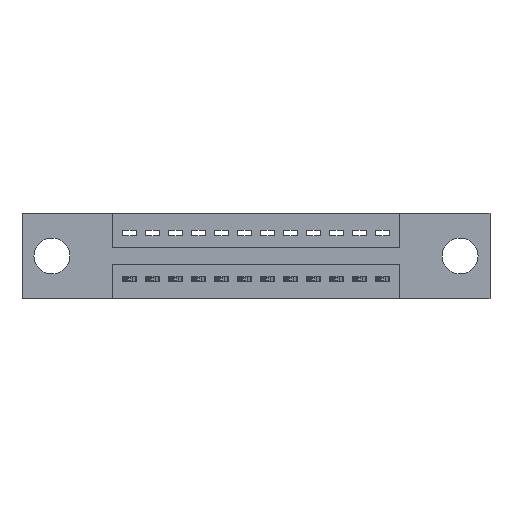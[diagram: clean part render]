
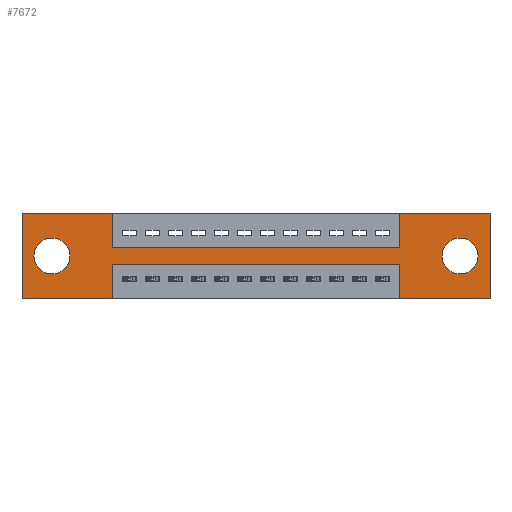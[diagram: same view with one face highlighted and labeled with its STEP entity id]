
A CAD part, front view. The second image highlights one B-rep face of the part: STEP entity #7672.
In plain terms, the highlighted planar face has unit normal (0, -1, 0).
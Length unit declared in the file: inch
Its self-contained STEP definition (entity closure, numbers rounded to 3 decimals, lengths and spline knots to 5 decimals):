
#318 = ORIENTED_EDGE ( 'NONE', *, *, #12914, .F. ) ;
#356 = VECTOR ( 'NONE', #7961, 39.37008 ) ;
#487 = EDGE_CURVE ( 'NONE', #9117, #1212, #12375, .T. ) ;
#604 = DIRECTION ( 'NONE',  ( -1., 0., 0. ) ) ;
#720 = ORIENTED_EDGE ( 'NONE', *, *, #12855, .F. ) ;
#855 = EDGE_CURVE ( 'NONE', #6111, #11537, #11433, .T. ) ;
#1012 = VECTOR ( 'NONE', #604, 39.37008 ) ;
#1043 = PLANE ( 'NONE',  #3110 ) ;
#1212 = VERTEX_POINT ( 'NONE', #1814 ) ;
#1356 = VECTOR ( 'NONE', #6458, 39.37008 ) ;
#1400 = DIRECTION ( 'NONE',  ( 0., 1., 0. ) ) ;
#1408 = ORIENTED_EDGE ( 'NONE', *, *, #5395, .F. ) ;
#1462 = CARTESIAN_POINT ( 'NONE',  ( 0., 0., 0. ) ) ;
#1665 = DIRECTION ( 'NONE',  ( 1., 0., 0. ) ) ;
#1699 = VECTOR ( 'NONE', #12983, 39.37008 ) ;
#1769 = EDGE_LOOP ( 'NONE', ( #11584, #6691 ) ) ;
#1786 = CARTESIAN_POINT ( 'NONE',  ( 1.6425, 0., 0. ) ) ;
#1814 = CARTESIAN_POINT ( 'NONE',  ( 1.6425, 0., -0.22 ) ) ;
#1876 = CARTESIAN_POINT ( 'NONE',  ( 1.905, 0., -0.263 ) ) ;
#1908 = VERTEX_POINT ( 'NONE', #6651 ) ;
#2068 = CARTESIAN_POINT ( 'NONE',  ( 0., 0., -0.37 ) ) ;
#2080 = EDGE_CURVE ( 'NONE', #7362, #10006, #7179, .T. ) ;
#2189 = CIRCLE ( 'NONE', #7160, 0.078 ) ;
#2197 = ORIENTED_EDGE ( 'NONE', *, *, #4360, .F. ) ;
#2454 = LINE ( 'NONE', #3017, #1699 ) ;
#2482 = EDGE_CURVE ( 'NONE', #6165, #11500, #4491, .T. ) ;
#2590 = EDGE_LOOP ( 'NONE', ( #10549, #720, #6742, #1408, #318, #6607, #2197, #4417, #5114, #8214, #8763, #4503 ) ) ;
#2599 = CARTESIAN_POINT ( 'NONE',  ( 0.13, 0., -0.107 ) ) ;
#2785 = DIRECTION ( 'NONE',  ( 0., 0., 1. ) ) ;
#2831 = DIRECTION ( 'NONE',  ( 0., 1., 0. ) ) ;
#2920 = VERTEX_POINT ( 'NONE', #3381 ) ;
#3017 = CARTESIAN_POINT ( 'NONE',  ( 0.3925, 0., -0.37 ) ) ;
#3110 = AXIS2_PLACEMENT_3D ( 'NONE', #2068, #6134, #8131 ) ;
#3120 = AXIS2_PLACEMENT_3D ( 'NONE', #12796, #2831, #2785 ) ;
#3379 = FACE_OUTER_BOUND ( 'NONE', #2590, .T. ) ;
#3381 = CARTESIAN_POINT ( 'NONE',  ( 2.035, 0., -0.37 ) ) ;
#3842 = ORIENTED_EDGE ( 'NONE', *, *, #10488, .T. ) ;
#3873 = VECTOR ( 'NONE', #1665, 39.37008 ) ;
#3937 = DIRECTION ( 'NONE',  ( 0., 0., -1. ) ) ;
#4031 = CARTESIAN_POINT ( 'NONE',  ( 0.3925, 0., -0.22 ) ) ;
#4063 = EDGE_CURVE ( 'NONE', #4259, #1908, #7414, .T. ) ;
#4072 = CARTESIAN_POINT ( 'NONE',  ( 2.035, 0., 0. ) ) ;
#4089 = CARTESIAN_POINT ( 'NONE',  ( 0., 0., -0.37 ) ) ;
#4112 = LINE ( 'NONE', #12458, #1356 ) ;
#4259 = VERTEX_POINT ( 'NONE', #6526 ) ;
#4360 = EDGE_CURVE ( 'NONE', #11500, #7362, #11028, .T. ) ;
#4417 = ORIENTED_EDGE ( 'NONE', *, *, #2482, .F. ) ;
#4491 = LINE ( 'NONE', #12496, #3873 ) ;
#4503 = ORIENTED_EDGE ( 'NONE', *, *, #6720, .F. ) ;
#4535 = LINE ( 'NONE', #4072, #10818 ) ;
#4577 = CARTESIAN_POINT ( 'NONE',  ( 2.035, 0., 0. ) ) ;
#4677 = AXIS2_PLACEMENT_3D ( 'NONE', #5333, #1400, #12327 ) ;
#4707 = DIRECTION ( 'NONE',  ( 0., 0., 1. ) ) ;
#4844 = EDGE_CURVE ( 'NONE', #11537, #6111, #2189, .T. ) ;
#4854 = LINE ( 'NONE', #4031, #356 ) ;
#4955 = CARTESIAN_POINT ( 'NONE',  ( 0.13, 0., -0.185 ) ) ;
#5114 = ORIENTED_EDGE ( 'NONE', *, *, #11751, .F. ) ;
#5144 = FACE_BOUND ( 'NONE', #11985, .T. ) ;
#5333 = CARTESIAN_POINT ( 'NONE',  ( 1.905, 0., -0.185 ) ) ;
#5380 = VECTOR ( 'NONE', #10986, 39.37008 ) ;
#5395 = EDGE_CURVE ( 'NONE', #2920, #9117, #11801, .T. ) ;
#5415 = VECTOR ( 'NONE', #5840, 39.37008 ) ;
#5786 = CARTESIAN_POINT ( 'NONE',  ( 1.6425, 0., -0.15 ) ) ;
#5800 = DIRECTION ( 'NONE',  ( 1., 0., 0. ) ) ;
#5840 = DIRECTION ( 'NONE',  ( 1., 0., 0. ) ) ;
#5864 = ORIENTED_EDGE ( 'NONE', *, *, #7198, .T. ) ;
#5935 = VECTOR ( 'NONE', #5800, 39.37008 ) ;
#5963 = CIRCLE ( 'NONE', #9448, 0.078 ) ;
#6034 = DIRECTION ( 'NONE',  ( 0., 0., 1. ) ) ;
#6111 = VERTEX_POINT ( 'NONE', #7629 ) ;
#6134 = DIRECTION ( 'NONE',  ( 0., -1., 0. ) ) ;
#6165 = VERTEX_POINT ( 'NONE', #6584 ) ;
#6458 = DIRECTION ( 'NONE',  ( 0., 0., 1. ) ) ;
#6526 = CARTESIAN_POINT ( 'NONE',  ( 0., 0., 0. ) ) ;
#6584 = CARTESIAN_POINT ( 'NONE',  ( 0.3925, 0., -0.15 ) ) ;
#6607 = ORIENTED_EDGE ( 'NONE', *, *, #2080, .F. ) ;
#6651 = CARTESIAN_POINT ( 'NONE',  ( 0.3925, 0., 0. ) ) ;
#6691 = ORIENTED_EDGE ( 'NONE', *, *, #855, .T. ) ;
#6720 = EDGE_CURVE ( 'NONE', #10745, #7590, #8146, .T. ) ;
#6742 = ORIENTED_EDGE ( 'NONE', *, *, #487, .F. ) ;
#7160 = AXIS2_PLACEMENT_3D ( 'NONE', #4955, #8895, #6034 ) ;
#7179 = LINE ( 'NONE', #8079, #5935 ) ;
#7198 = EDGE_CURVE ( 'NONE', #10978, #10078, #5963, .T. ) ;
#7362 = VERTEX_POINT ( 'NONE', #8374 ) ;
#7414 = LINE ( 'NONE', #1462, #5415 ) ;
#7509 = VECTOR ( 'NONE', #4707, 39.37008 ) ;
#7590 = VERTEX_POINT ( 'NONE', #7965 ) ;
#7629 = CARTESIAN_POINT ( 'NONE',  ( 0.13, 0., -0.263 ) ) ;
#7672 = ADVANCED_FACE ( 'NONE', ( #5144, #12506, #3379 ), #1043, .T. ) ;
#7961 = DIRECTION ( 'NONE',  ( -1., 0., 0. ) ) ;
#7965 = CARTESIAN_POINT ( 'NONE',  ( 0., 0., -0.37 ) ) ;
#8056 = VECTOR ( 'NONE', #12950, 39.37008 ) ;
#8079 = CARTESIAN_POINT ( 'NONE',  ( 0., 0., 0. ) ) ;
#8131 = DIRECTION ( 'NONE',  ( 0., 0., -1. ) ) ;
#8146 = LINE ( 'NONE', #12529, #1012 ) ;
#8214 = ORIENTED_EDGE ( 'NONE', *, *, #4063, .F. ) ;
#8329 = CARTESIAN_POINT ( 'NONE',  ( 1.905, 0., -0.185 ) ) ;
#8374 = CARTESIAN_POINT ( 'NONE',  ( 1.6425, 0., 0. ) ) ;
#8587 = CARTESIAN_POINT ( 'NONE',  ( 1.6425, 0., -0.37 ) ) ;
#8763 = ORIENTED_EDGE ( 'NONE', *, *, #12027, .F. ) ;
#8895 = DIRECTION ( 'NONE',  ( 0., 1., 0. ) ) ;
#8987 = CARTESIAN_POINT ( 'NONE',  ( 0.3925, 0., 0. ) ) ;
#9117 = VERTEX_POINT ( 'NONE', #11061 ) ;
#9173 = DIRECTION ( 'NONE',  ( 0., 0., -1. ) ) ;
#9441 = LINE ( 'NONE', #8987, #9593 ) ;
#9448 = AXIS2_PLACEMENT_3D ( 'NONE', #8329, #12222, #9173 ) ;
#9593 = VECTOR ( 'NONE', #3937, 39.37008 ) ;
#10006 = VERTEX_POINT ( 'NONE', #4577 ) ;
#10078 = VERTEX_POINT ( 'NONE', #10102 ) ;
#10102 = CARTESIAN_POINT ( 'NONE',  ( 1.905, 0., -0.107 ) ) ;
#10488 = EDGE_CURVE ( 'NONE', #10078, #10978, #12583, .T. ) ;
#10549 = ORIENTED_EDGE ( 'NONE', *, *, #11739, .F. ) ;
#10745 = VERTEX_POINT ( 'NONE', #12398 ) ;
#10764 = CARTESIAN_POINT ( 'NONE',  ( 0.3925, 0., -0.22 ) ) ;
#10818 = VECTOR ( 'NONE', #12238, 39.37008 ) ;
#10978 = VERTEX_POINT ( 'NONE', #1876 ) ;
#10986 = DIRECTION ( 'NONE',  ( -1., 0., 0. ) ) ;
#11028 = LINE ( 'NONE', #1786, #8056 ) ;
#11061 = CARTESIAN_POINT ( 'NONE',  ( 1.6425, 0., -0.37 ) ) ;
#11433 = CIRCLE ( 'NONE', #3120, 0.078 ) ;
#11500 = VERTEX_POINT ( 'NONE', #5786 ) ;
#11537 = VERTEX_POINT ( 'NONE', #2599 ) ;
#11577 = VERTEX_POINT ( 'NONE', #10764 ) ;
#11584 = ORIENTED_EDGE ( 'NONE', *, *, #4844, .T. ) ;
#11739 = EDGE_CURVE ( 'NONE', #11577, #10745, #2454, .T. ) ;
#11751 = EDGE_CURVE ( 'NONE', #1908, #6165, #9441, .T. ) ;
#11801 = LINE ( 'NONE', #4089, #5380 ) ;
#11985 = EDGE_LOOP ( 'NONE', ( #3842, #5864 ) ) ;
#12027 = EDGE_CURVE ( 'NONE', #7590, #4259, #4112, .T. ) ;
#12222 = DIRECTION ( 'NONE',  ( 0., 1., 0. ) ) ;
#12238 = DIRECTION ( 'NONE',  ( 0., 0., -1. ) ) ;
#12327 = DIRECTION ( 'NONE',  ( 0., 0., -1. ) ) ;
#12375 = LINE ( 'NONE', #8587, #7509 ) ;
#12398 = CARTESIAN_POINT ( 'NONE',  ( 0.3925, 0., -0.37 ) ) ;
#12458 = CARTESIAN_POINT ( 'NONE',  ( 0., 0., 0. ) ) ;
#12496 = CARTESIAN_POINT ( 'NONE',  ( 0.3925, 0., -0.15 ) ) ;
#12506 = FACE_BOUND ( 'NONE', #1769, .T. ) ;
#12529 = CARTESIAN_POINT ( 'NONE',  ( 0., 0., -0.37 ) ) ;
#12583 = CIRCLE ( 'NONE', #4677, 0.078 ) ;
#12796 = CARTESIAN_POINT ( 'NONE',  ( 0.13, 0., -0.185 ) ) ;
#12855 = EDGE_CURVE ( 'NONE', #1212, #11577, #4854, .T. ) ;
#12914 = EDGE_CURVE ( 'NONE', #10006, #2920, #4535, .T. ) ;
#12950 = DIRECTION ( 'NONE',  ( 0., 0., 1. ) ) ;
#12983 = DIRECTION ( 'NONE',  ( 0., 0., -1. ) ) ;
